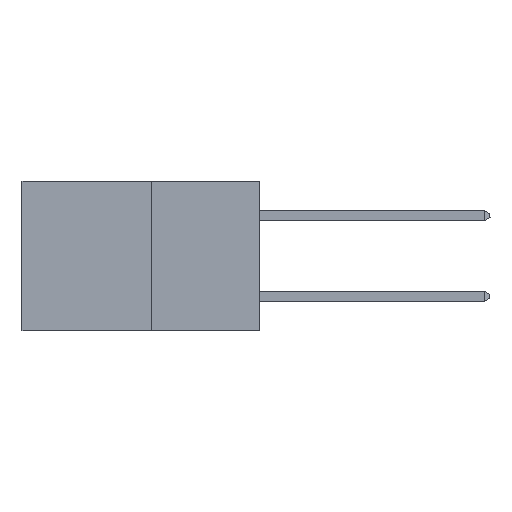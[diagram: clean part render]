
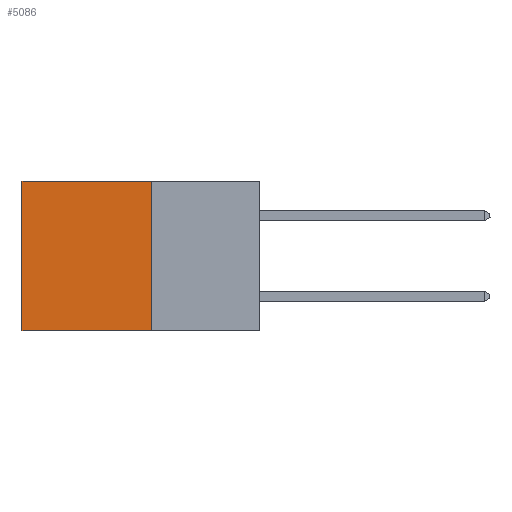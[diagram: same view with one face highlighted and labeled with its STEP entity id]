
A CAD part, left-side view. The second image highlights one B-rep face of the part: STEP entity #5086.
In plain terms, the highlighted planar face has unit normal (-1, 0, 0).
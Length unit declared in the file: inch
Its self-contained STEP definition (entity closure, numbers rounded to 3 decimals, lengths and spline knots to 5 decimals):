
#368 = VECTOR ( 'NONE', #25477, 39.37008 ) ;
#1196 = EDGE_LOOP ( 'NONE', ( #7634, #1951, #26753, #4936 ) ) ;
#1576 = LINE ( 'NONE', #18844, #8487 ) ;
#1951 = ORIENTED_EDGE ( 'NONE', *, *, #12598, .F. ) ;
#3865 = CARTESIAN_POINT ( 'NONE',  ( 0.277, 0.27, -0.37 ) ) ;
#4411 = CARTESIAN_POINT ( 'NONE',  ( 0.277, 0.27, -0.37 ) ) ;
#4680 = VECTOR ( 'NONE', #7003, 39.37008 ) ;
#4936 = ORIENTED_EDGE ( 'NONE', *, *, #5248, .T. ) ;
#5067 = EDGE_CURVE ( 'NONE', #12797, #15909, #27833, .T. ) ;
#5086 = ADVANCED_FACE ( 'NONE', ( #21085 ), #32640, .F. ) ;
#5248 = EDGE_CURVE ( 'NONE', #23860, #12797, #1576, .T. ) ;
#7003 = DIRECTION ( 'NONE',  ( 0., 1., 0. ) ) ;
#7634 = ORIENTED_EDGE ( 'NONE', *, *, #5067, .T. ) ;
#8218 = EDGE_CURVE ( 'NONE', #23860, #13927, #13643, .T. ) ;
#8487 = VECTOR ( 'NONE', #18204, 39.37008 ) ;
#9942 = CARTESIAN_POINT ( 'NONE',  ( 0.277, 0.27, -0.37 ) ) ;
#10819 = CARTESIAN_POINT ( 'NONE',  ( 0.277, 0.59, -0.37 ) ) ;
#11562 = LINE ( 'NONE', #4411, #4680 ) ;
#12598 = EDGE_CURVE ( 'NONE', #13927, #15909, #11562, .T. ) ;
#12797 = VERTEX_POINT ( 'NONE', #20717 ) ;
#13267 = CARTESIAN_POINT ( 'NONE',  ( 0.277, 0.27, 0. ) ) ;
#13643 = LINE ( 'NONE', #3865, #28069 ) ;
#13927 = VERTEX_POINT ( 'NONE', #9942 ) ;
#15211 = CARTESIAN_POINT ( 'NONE',  ( 0.277, 0.59, -0.37 ) ) ;
#15909 = VERTEX_POINT ( 'NONE', #15211 ) ;
#18204 = DIRECTION ( 'NONE',  ( 0., 1., 0. ) ) ;
#18844 = CARTESIAN_POINT ( 'NONE',  ( 0.277, 0.27, 0. ) ) ;
#20717 = CARTESIAN_POINT ( 'NONE',  ( 0.277, 0.59, 0. ) ) ;
#21085 = FACE_OUTER_BOUND ( 'NONE', #1196, .T. ) ;
#21988 = DIRECTION ( 'NONE',  ( 0., 0., -1. ) ) ;
#22534 = AXIS2_PLACEMENT_3D ( 'NONE', #24786, #29250, #27093 ) ;
#23860 = VERTEX_POINT ( 'NONE', #13267 ) ;
#24786 = CARTESIAN_POINT ( 'NONE',  ( 0.277, 0.27, -0.37 ) ) ;
#25477 = DIRECTION ( 'NONE',  ( 0., 0., -1. ) ) ;
#26753 = ORIENTED_EDGE ( 'NONE', *, *, #8218, .F. ) ;
#27093 = DIRECTION ( 'NONE',  ( 0., 0., -1. ) ) ;
#27833 = LINE ( 'NONE', #10819, #368 ) ;
#28069 = VECTOR ( 'NONE', #21988, 39.37008 ) ;
#29250 = DIRECTION ( 'NONE',  ( 1., 0., 0. ) ) ;
#32640 = PLANE ( 'NONE',  #22534 ) ;
